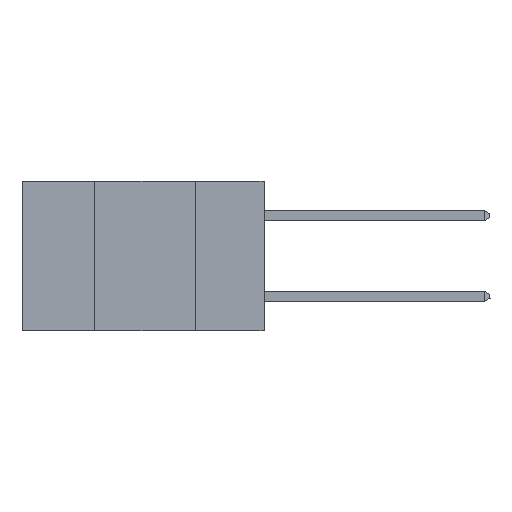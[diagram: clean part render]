
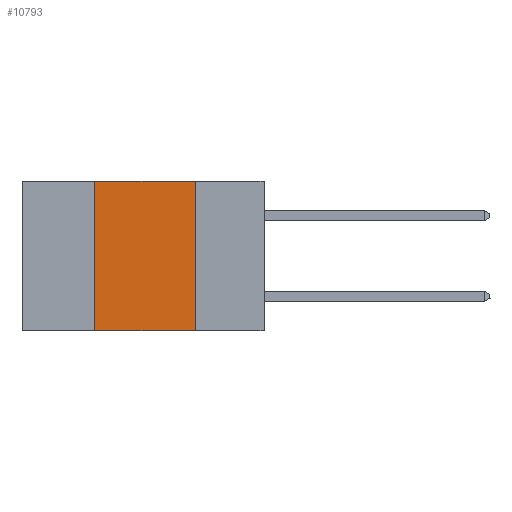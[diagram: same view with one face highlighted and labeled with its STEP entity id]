
A CAD part, left-side view. The second image highlights one B-rep face of the part: STEP entity #10793.
In plain terms, the highlighted planar face has unit normal (-1, 0, 0).
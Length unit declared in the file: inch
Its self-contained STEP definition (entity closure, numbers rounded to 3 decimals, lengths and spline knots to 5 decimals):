
#24 = ORIENTED_EDGE ( 'NONE', *, *, #5490, .F. ) ;
#142 = ORIENTED_EDGE ( 'NONE', *, *, #18577, .F. ) ;
#1029 = VECTOR ( 'NONE', #22326, 39.37008 ) ;
#1542 = AXIS2_PLACEMENT_3D ( 'NONE', #12293, #17392, #17555 ) ;
#1869 = VERTEX_POINT ( 'NONE', #26366 ) ;
#2170 = CARTESIAN_POINT ( 'NONE',  ( 0., 0.6, 0. ) ) ;
#2815 = CARTESIAN_POINT ( 'NONE',  ( 0., 0.17, 0. ) ) ;
#3617 = CARTESIAN_POINT ( 'NONE',  ( 0., 0.6, -0.37 ) ) ;
#4033 = VERTEX_POINT ( 'NONE', #20494 ) ;
#5216 = VECTOR ( 'NONE', #21528, 39.37008 ) ;
#5490 = EDGE_CURVE ( 'NONE', #13775, #1869, #23709, .T. ) ;
#5785 = EDGE_CURVE ( 'NONE', #1869, #9578, #10386, .T. ) ;
#5877 = DIRECTION ( 'NONE',  ( 0., -1., 0. ) ) ;
#9524 = VECTOR ( 'NONE', #5877, 39.37008 ) ;
#9578 = VERTEX_POINT ( 'NONE', #2815 ) ;
#10386 = LINE ( 'NONE', #2170, #5216 ) ;
#10793 = ADVANCED_FACE ( 'NONE', ( #11553 ), #12976, .F. ) ;
#11235 = EDGE_LOOP ( 'NONE', ( #142, #24604, #24, #15930 ) ) ;
#11553 = FACE_OUTER_BOUND ( 'NONE', #11235, .T. ) ;
#12293 = CARTESIAN_POINT ( 'NONE',  ( 0., 0.6, 0. ) ) ;
#12976 = PLANE ( 'NONE',  #1542 ) ;
#13015 = VECTOR ( 'NONE', #14625, 39.37008 ) ;
#13775 = VERTEX_POINT ( 'NONE', #26758 ) ;
#14625 = DIRECTION ( 'NONE',  ( 0., 0., -1. ) ) ;
#15930 = ORIENTED_EDGE ( 'NONE', *, *, #19137, .T. ) ;
#17392 = DIRECTION ( 'NONE',  ( 1., 0., 0. ) ) ;
#17555 = DIRECTION ( 'NONE',  ( 0., 0., -1. ) ) ;
#18577 = EDGE_CURVE ( 'NONE', #9578, #4033, #23895, .T. ) ;
#19137 = EDGE_CURVE ( 'NONE', #13775, #4033, #26792, .T. ) ;
#20494 = CARTESIAN_POINT ( 'NONE',  ( 0., 0.17, -0.37 ) ) ;
#21528 = DIRECTION ( 'NONE',  ( 0., -1., 0. ) ) ;
#22326 = DIRECTION ( 'NONE',  ( 0., 0., 1. ) ) ;
#23709 = LINE ( 'NONE', #24031, #1029 ) ;
#23895 = LINE ( 'NONE', #27526, #13015 ) ;
#24031 = CARTESIAN_POINT ( 'NONE',  ( 0., 0.42, 0. ) ) ;
#24604 = ORIENTED_EDGE ( 'NONE', *, *, #5785, .F. ) ;
#26366 = CARTESIAN_POINT ( 'NONE',  ( 0., 0.42, 0. ) ) ;
#26758 = CARTESIAN_POINT ( 'NONE',  ( 0., 0.42, -0.37 ) ) ;
#26792 = LINE ( 'NONE', #3617, #9524 ) ;
#27526 = CARTESIAN_POINT ( 'NONE',  ( 0., 0.17, 0. ) ) ;
